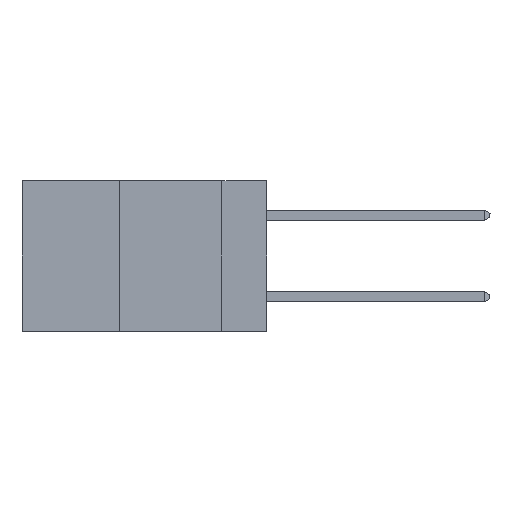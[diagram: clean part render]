
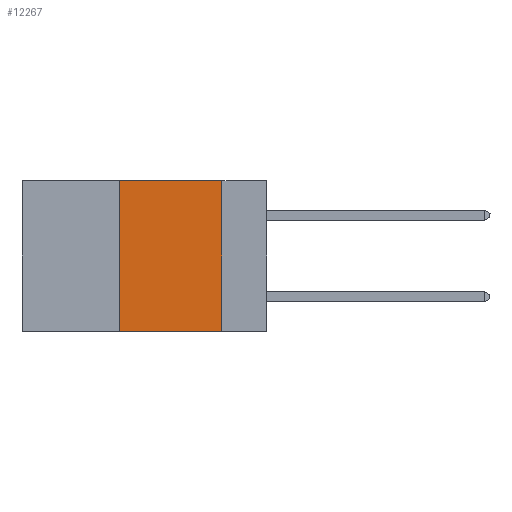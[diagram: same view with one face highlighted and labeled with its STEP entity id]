
A CAD part, left-side view. The second image highlights one B-rep face of the part: STEP entity #12267.
In plain terms, the highlighted planar face has unit normal (-1, 0, 0).
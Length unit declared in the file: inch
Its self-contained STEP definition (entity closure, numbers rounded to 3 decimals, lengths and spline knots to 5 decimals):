
#10 = VERTEX_POINT ( 'NONE', #23235 ) ;
#659 = EDGE_CURVE ( 'NONE', #22300, #840, #1033, .T. ) ;
#785 = EDGE_LOOP ( 'NONE', ( #13374, #14827, #16223, #1764 ) ) ;
#840 = VERTEX_POINT ( 'NONE', #1398 ) ;
#1033 = LINE ( 'NONE', #13921, #14285 ) ;
#1398 = CARTESIAN_POINT ( 'NONE',  ( 0., 0.11, 0. ) ) ;
#1764 = ORIENTED_EDGE ( 'NONE', *, *, #22486, .T. ) ;
#2523 = DIRECTION ( 'NONE',  ( 0., 0., -1. ) ) ;
#3766 = LINE ( 'NONE', #20389, #14077 ) ;
#4085 = LINE ( 'NONE', #11782, #15788 ) ;
#4523 = PLANE ( 'NONE',  #17058 ) ;
#7151 = DIRECTION ( 'NONE',  ( 0., 0., 1. ) ) ;
#8045 = EDGE_CURVE ( 'NONE', #840, #10, #4085, .T. ) ;
#8276 = CARTESIAN_POINT ( 'NONE',  ( 0., 0.36, 0. ) ) ;
#10666 = LINE ( 'NONE', #12355, #15490 ) ;
#11742 = DIRECTION ( 'NONE',  ( 1., 0., 0. ) ) ;
#11782 = CARTESIAN_POINT ( 'NONE',  ( 0., 0.11, 0. ) ) ;
#12267 = ADVANCED_FACE ( 'NONE', ( #17745 ), #4523, .F. ) ;
#12355 = CARTESIAN_POINT ( 'NONE',  ( 0., 0.6, -0.37 ) ) ;
#12592 = DIRECTION ( 'NONE',  ( 0., -1., 0. ) ) ;
#13374 = ORIENTED_EDGE ( 'NONE', *, *, #8045, .F. ) ;
#13921 = CARTESIAN_POINT ( 'NONE',  ( 0., 0.6, 0. ) ) ;
#14010 = CARTESIAN_POINT ( 'NONE',  ( 0., 0.36, -0.37 ) ) ;
#14077 = VECTOR ( 'NONE', #7151, 39.37008 ) ;
#14285 = VECTOR ( 'NONE', #15606, 39.37008 ) ;
#14827 = ORIENTED_EDGE ( 'NONE', *, *, #659, .F. ) ;
#15490 = VECTOR ( 'NONE', #12592, 39.37008 ) ;
#15606 = DIRECTION ( 'NONE',  ( 0., -1., 0. ) ) ;
#15788 = VECTOR ( 'NONE', #2523, 39.37008 ) ;
#16223 = ORIENTED_EDGE ( 'NONE', *, *, #16804, .F. ) ;
#16804 = EDGE_CURVE ( 'NONE', #17836, #22300, #3766, .T. ) ;
#17058 = AXIS2_PLACEMENT_3D ( 'NONE', #20889, #11742, #21251 ) ;
#17745 = FACE_OUTER_BOUND ( 'NONE', #785, .T. ) ;
#17836 = VERTEX_POINT ( 'NONE', #14010 ) ;
#20389 = CARTESIAN_POINT ( 'NONE',  ( 0., 0.36, 0. ) ) ;
#20889 = CARTESIAN_POINT ( 'NONE',  ( 0., 0.6, 0. ) ) ;
#21251 = DIRECTION ( 'NONE',  ( 0., 0., -1. ) ) ;
#22300 = VERTEX_POINT ( 'NONE', #8276 ) ;
#22486 = EDGE_CURVE ( 'NONE', #17836, #10, #10666, .T. ) ;
#23235 = CARTESIAN_POINT ( 'NONE',  ( 0., 0.11, -0.37 ) ) ;
